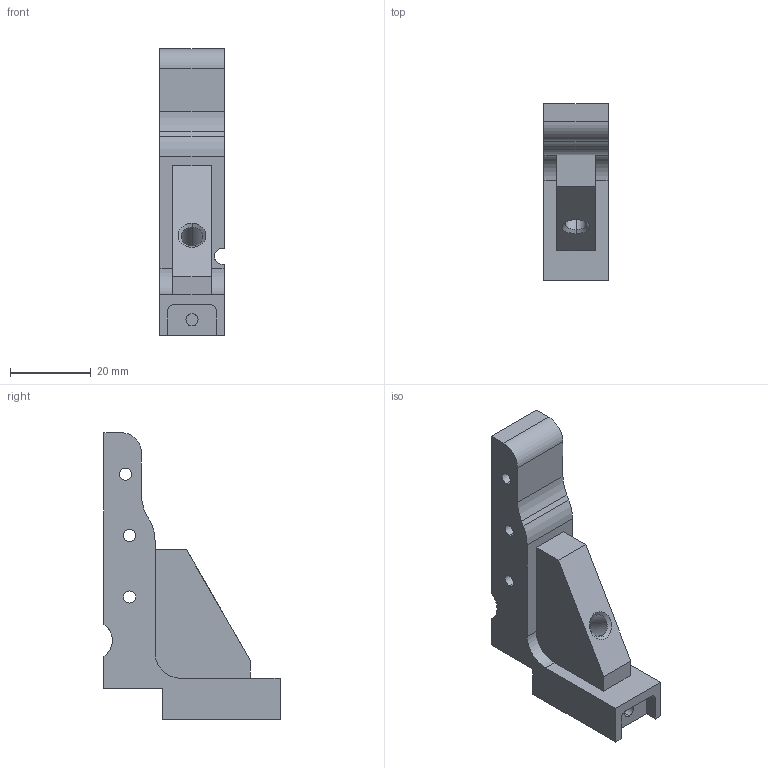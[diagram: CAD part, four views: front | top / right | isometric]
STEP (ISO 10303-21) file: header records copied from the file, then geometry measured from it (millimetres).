
FILE_DESCRIPTION (( 'STEP AP214' ), '1' );
FILE_NAME ('Thunderbolt_Grip_Part.STEP', '2021-09-12T03:49:29', ( '' ), ( '' ), 'SwSTEP 2.0', 'SolidWorks 2020', '' );
FILE_SCHEMA (( 'AUTOMOTIVE_DESIGN' ));
Length unit declared in the file: millimetre
Products named in the file (1): Thunderbolt_Grip_Part
Bounding box: 15.88 x 43.56 x 70.9 mm (x, y, z)
Volume: 17602.8 mm3; surface area: 8151.4 mm2
Topology: 1 solids, 1 shells, 75 faces, 211 edges, 140 vertices
Faces by surface type: plane 45, cylinder 28, cone 2
Entity records: 2514 total; most frequent: CARTESIAN_POINT 472, ORIENTED_EDGE 422, DIRECTION 410, EDGE_CURVE 211, LINE 150, VECTOR 150, VERTEX_POINT 140, AXIS2_PLACEMENT_3D 130
